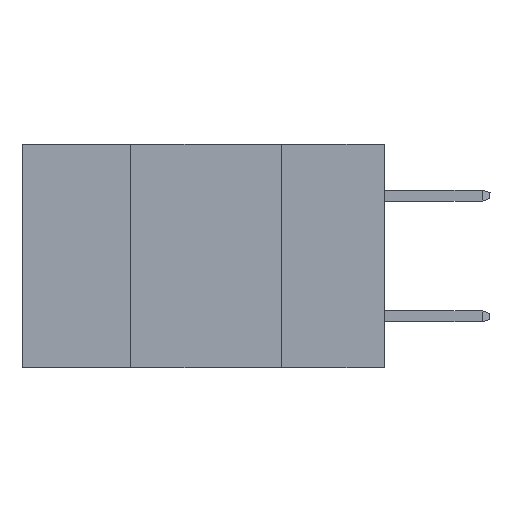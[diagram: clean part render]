
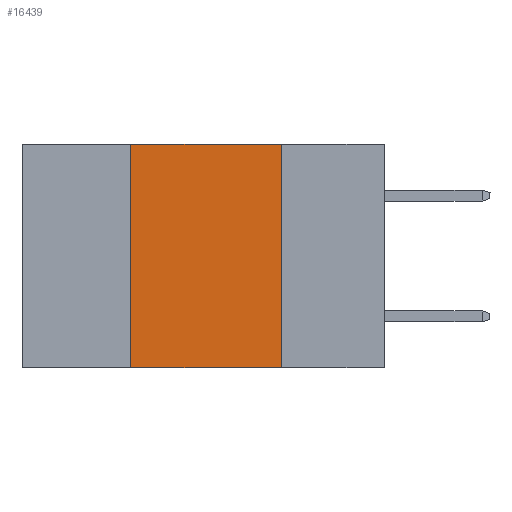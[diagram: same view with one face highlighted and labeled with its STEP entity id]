
A CAD part, left-side view. The second image highlights one B-rep face of the part: STEP entity #16439.
In plain terms, the highlighted planar face has unit normal (-1, 0, 0).
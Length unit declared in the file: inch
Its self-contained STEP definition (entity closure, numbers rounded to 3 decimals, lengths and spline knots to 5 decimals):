
#460 = LINE ( 'NONE', #22845, #18647 ) ;
#773 = ORIENTED_EDGE ( 'NONE', *, *, #17384, .T. ) ;
#1276 = CARTESIAN_POINT ( 'NONE',  ( 0., 0.17, 0. ) ) ;
#1370 = CARTESIAN_POINT ( 'NONE',  ( 0., 0.42, 0. ) ) ;
#1520 = ORIENTED_EDGE ( 'NONE', *, *, #8950, .F. ) ;
#2785 = CARTESIAN_POINT ( 'NONE',  ( 0., 0.17, -0.37 ) ) ;
#3002 = VECTOR ( 'NONE', #19629, 39.37008 ) ;
#3990 = EDGE_CURVE ( 'NONE', #16924, #13405, #16351, .T. ) ;
#4325 = AXIS2_PLACEMENT_3D ( 'NONE', #15011, #10681, #23325 ) ;
#5968 = DIRECTION ( 'NONE',  ( 0., -1., 0. ) ) ;
#6214 = LINE ( 'NONE', #17427, #3002 ) ;
#7894 = VECTOR ( 'NONE', #5968, 39.37008 ) ;
#7930 = ORIENTED_EDGE ( 'NONE', *, *, #3990, .F. ) ;
#8950 = EDGE_CURVE ( 'NONE', #19142, #16924, #15838, .T. ) ;
#9917 = FACE_OUTER_BOUND ( 'NONE', #25474, .T. ) ;
#10681 = DIRECTION ( 'NONE',  ( 1., 0., 0. ) ) ;
#11132 = EDGE_CURVE ( 'NONE', #13405, #21759, #6214, .T. ) ;
#12010 = DIRECTION ( 'NONE',  ( 0., 0., 1. ) ) ;
#13405 = VERTEX_POINT ( 'NONE', #1276 ) ;
#13868 = CARTESIAN_POINT ( 'NONE',  ( 0., 0.42, 0. ) ) ;
#14524 = DIRECTION ( 'NONE',  ( 0., -1., 0. ) ) ;
#15011 = CARTESIAN_POINT ( 'NONE',  ( 0., 0.6, 0. ) ) ;
#15838 = LINE ( 'NONE', #1370, #16146 ) ;
#16146 = VECTOR ( 'NONE', #12010, 39.37008 ) ;
#16351 = LINE ( 'NONE', #18537, #7894 ) ;
#16439 = ADVANCED_FACE ( 'NONE', ( #9917 ), #19263, .F. ) ;
#16924 = VERTEX_POINT ( 'NONE', #13868 ) ;
#17210 = CARTESIAN_POINT ( 'NONE',  ( 0., 0.42, -0.37 ) ) ;
#17384 = EDGE_CURVE ( 'NONE', #19142, #21759, #460, .T. ) ;
#17427 = CARTESIAN_POINT ( 'NONE',  ( 0., 0.17, 0. ) ) ;
#18537 = CARTESIAN_POINT ( 'NONE',  ( 0., 0.6, 0. ) ) ;
#18647 = VECTOR ( 'NONE', #14524, 39.37008 ) ;
#19142 = VERTEX_POINT ( 'NONE', #17210 ) ;
#19263 = PLANE ( 'NONE',  #4325 ) ;
#19629 = DIRECTION ( 'NONE',  ( 0., 0., -1. ) ) ;
#21759 = VERTEX_POINT ( 'NONE', #2785 ) ;
#22308 = ORIENTED_EDGE ( 'NONE', *, *, #11132, .F. ) ;
#22845 = CARTESIAN_POINT ( 'NONE',  ( 0., 0.6, -0.37 ) ) ;
#23325 = DIRECTION ( 'NONE',  ( 0., 0., -1. ) ) ;
#25474 = EDGE_LOOP ( 'NONE', ( #22308, #7930, #1520, #773 ) ) ;
